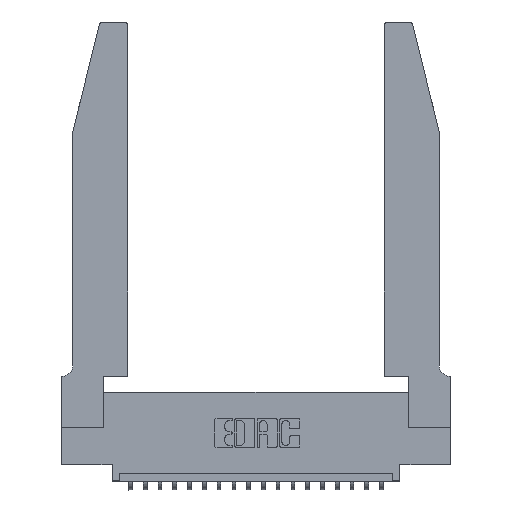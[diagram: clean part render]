
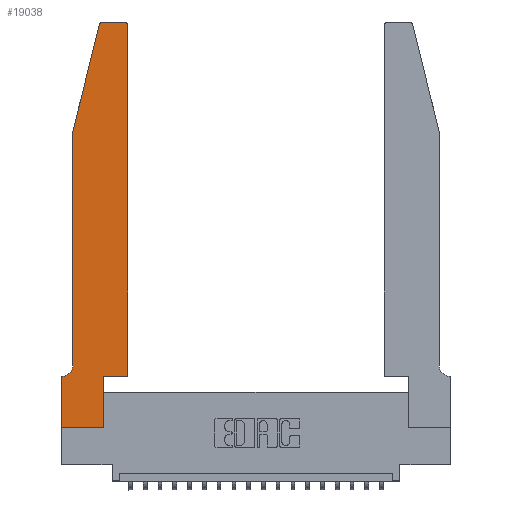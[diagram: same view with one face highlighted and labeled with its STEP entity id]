
A CAD part, top view. The second image highlights one B-rep face of the part: STEP entity #19038.
In plain terms, the highlighted planar face has unit normal (0, 0, 1).
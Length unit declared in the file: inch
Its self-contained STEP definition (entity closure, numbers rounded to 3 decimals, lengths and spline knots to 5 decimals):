
#1 = EDGE_CURVE ( 'NONE', #4615, #11518, #21165, .T. ) ;
#22 = CARTESIAN_POINT ( 'NONE',  ( 0.0755, 0.42, 0.37 ) ) ;
#1192 = DIRECTION ( 'NONE',  ( 1., 0., 0. ) ) ;
#1444 = CARTESIAN_POINT ( 'NONE',  ( 0., 0., 0.37 ) ) ;
#1651 = DIRECTION ( 'NONE',  ( 0., 0., 1. ) ) ;
#1704 = ORIENTED_EDGE ( 'NONE', *, *, #9884, .T. ) ;
#2663 = VECTOR ( 'NONE', #19163, 39.37008 ) ;
#2998 = CARTESIAN_POINT ( 'NONE',  ( 0.0755, 0.35, 0.37 ) ) ;
#3205 = DIRECTION ( 'NONE',  ( -1., 0., 0. ) ) ;
#3236 = EDGE_CURVE ( 'NONE', #10252, #7040, #8231, .T. ) ;
#3358 = CARTESIAN_POINT ( 'NONE',  ( 0., 0.35, 0.37 ) ) ;
#3461 = DIRECTION ( 'NONE',  ( 0., 0., 1. ) ) ;
#3543 = DIRECTION ( 'NONE',  ( 0., 0., 1. ) ) ;
#3619 = VERTEX_POINT ( 'NONE', #20377 ) ;
#4118 = AXIS2_PLACEMENT_3D ( 'NONE', #6324, #14975, #18029 ) ;
#4215 = VECTOR ( 'NONE', #3205, 39.37008 ) ;
#4345 = AXIS2_PLACEMENT_3D ( 'NONE', #15096, #3461, #5028 ) ;
#4615 = VERTEX_POINT ( 'NONE', #22 ) ;
#4709 = VERTEX_POINT ( 'NONE', #20488 ) ;
#4752 = DIRECTION ( 'NONE',  ( 0., -1., 0. ) ) ;
#4807 = ORIENTED_EDGE ( 'NONE', *, *, #6760, .T. ) ;
#5028 = DIRECTION ( 'NONE',  ( 1., 0., 0. ) ) ;
#5073 = DIRECTION ( 'NONE',  ( 1., 0., 0. ) ) ;
#5117 = ORIENTED_EDGE ( 'NONE', *, *, #3236, .T. ) ;
#5220 = VERTEX_POINT ( 'NONE', #20881 ) ;
#5966 = CARTESIAN_POINT ( 'NONE',  ( 0.2865, 0.35, 0.37 ) ) ;
#6016 = FACE_OUTER_BOUND ( 'NONE', #19877, .T. ) ;
#6113 = DIRECTION ( 'NONE',  ( 0., 1., 0. ) ) ;
#6208 = ORIENTED_EDGE ( 'NONE', *, *, #7324, .T. ) ;
#6324 = CARTESIAN_POINT ( 'NONE',  ( 0.0055, 0.42, 0.37 ) ) ;
#6427 = DIRECTION ( 'NONE',  ( -1., 0., 0. ) ) ;
#6599 = ORIENTED_EDGE ( 'NONE', *, *, #21737, .T. ) ;
#6621 = EDGE_CURVE ( 'NONE', #4709, #11150, #13332, .T. ) ;
#6627 = AXIS2_PLACEMENT_3D ( 'NONE', #8583, #3543, #20204 ) ;
#6760 = EDGE_CURVE ( 'NONE', #11150, #5220, #20127, .T. ) ;
#6766 = EDGE_CURVE ( 'NONE', #7576, #18585, #16740, .T. ) ;
#6931 = VECTOR ( 'NONE', #12697, 39.37008 ) ;
#7004 = VECTOR ( 'NONE', #1192, 39.37008 ) ;
#7040 = VERTEX_POINT ( 'NONE', #16041 ) ;
#7324 = EDGE_CURVE ( 'NONE', #18821, #4709, #19312, .T. ) ;
#7359 = LINE ( 'NONE', #5966, #11797 ) ;
#7439 = VECTOR ( 'NONE', #6427, 39.37008 ) ;
#7576 = VERTEX_POINT ( 'NONE', #8082 ) ;
#7864 = CARTESIAN_POINT ( 'NONE',  ( 0.4505, 0.35, 0.37 ) ) ;
#8082 = CARTESIAN_POINT ( 'NONE',  ( 0.284, 2.75, 0.37 ) ) ;
#8109 = VECTOR ( 'NONE', #14885, 39.37008 ) ;
#8231 = LINE ( 'NONE', #15295, #20787 ) ;
#8583 = CARTESIAN_POINT ( 'NONE',  ( 0.284, 2.72, 0.37 ) ) ;
#8804 = CARTESIAN_POINT ( 'NONE',  ( 0.4505, 2.72, 0.37 ) ) ;
#9005 = EDGE_CURVE ( 'NONE', #17906, #4615, #20296, .T. ) ;
#9147 = VECTOR ( 'NONE', #4752, 39.37008 ) ;
#9220 = CARTESIAN_POINT ( 'NONE',  ( 0.0755, 2., 0.37 ) ) ;
#9360 = CARTESIAN_POINT ( 'NONE',  ( 0.2865, 0.35, 0.37 ) ) ;
#9392 = LINE ( 'NONE', #18088, #9147 ) ;
#9553 = LINE ( 'NONE', #9220, #2663 ) ;
#9884 = EDGE_CURVE ( 'NONE', #5220, #7576, #21560, .T. ) ;
#10252 = VERTEX_POINT ( 'NONE', #1444 ) ;
#11150 = VERTEX_POINT ( 'NONE', #8804 ) ;
#11518 = VERTEX_POINT ( 'NONE', #20855 ) ;
#11589 = ORIENTED_EDGE ( 'NONE', *, *, #9005, .T. ) ;
#11640 = EDGE_CURVE ( 'NONE', #7040, #18821, #7359, .T. ) ;
#11797 = VECTOR ( 'NONE', #6113, 39.37008 ) ;
#12556 = CARTESIAN_POINT ( 'NONE',  ( 0.0755, 2., 0.37 ) ) ;
#12673 = LINE ( 'NONE', #2998, #7439 ) ;
#12697 = DIRECTION ( 'NONE',  ( 0., -1., 0. ) ) ;
#13332 = LINE ( 'NONE', #15124, #8109 ) ;
#13457 = DIRECTION ( 'NONE',  ( 1., 0., 0. ) ) ;
#13645 = ORIENTED_EDGE ( 'NONE', *, *, #6621, .T. ) ;
#13855 = CARTESIAN_POINT ( 'NONE',  ( 0.25487, 2.72718, 0.37 ) ) ;
#13914 = ORIENTED_EDGE ( 'NONE', *, *, #19600, .T. ) ;
#14885 = DIRECTION ( 'NONE',  ( 0., 1., 0. ) ) ;
#14975 = DIRECTION ( 'NONE',  ( 0., 0., -1. ) ) ;
#15064 = PLANE ( 'NONE',  #21667 ) ;
#15096 = CARTESIAN_POINT ( 'NONE',  ( 0.4205, 2.72, 0.37 ) ) ;
#15124 = CARTESIAN_POINT ( 'NONE',  ( 0.4505, 0.35, 0.37 ) ) ;
#15138 = CARTESIAN_POINT ( 'NONE',  ( 0.2605, 2.75, 0.37 ) ) ;
#15295 = CARTESIAN_POINT ( 'NONE',  ( 0., 0., 0.37 ) ) ;
#15922 = ORIENTED_EDGE ( 'NONE', *, *, #11640, .T. ) ;
#16041 = CARTESIAN_POINT ( 'NONE',  ( 0.2865, 0., 0.37 ) ) ;
#16740 = CIRCLE ( 'NONE', #6627, 0.03 ) ;
#16782 = EDGE_CURVE ( 'NONE', #11518, #3619, #12673, .T. ) ;
#17906 = VERTEX_POINT ( 'NONE', #18620 ) ;
#18029 = DIRECTION ( 'NONE',  ( -1., 0., 0. ) ) ;
#18088 = CARTESIAN_POINT ( 'NONE',  ( 0., 0., 0.37 ) ) ;
#18348 = ORIENTED_EDGE ( 'NONE', *, *, #16782, .T. ) ;
#18585 = VERTEX_POINT ( 'NONE', #13855 ) ;
#18620 = CARTESIAN_POINT ( 'NONE',  ( 0.0755, 2., 0.37 ) ) ;
#18821 = VERTEX_POINT ( 'NONE', #9360 ) ;
#19038 = ADVANCED_FACE ( 'NONE', ( #6016 ), #15064, .T. ) ;
#19163 = DIRECTION ( 'NONE',  ( -0.239, -0.971, 0. ) ) ;
#19312 = LINE ( 'NONE', #7864, #7004 ) ;
#19600 = EDGE_CURVE ( 'NONE', #3619, #10252, #9392, .T. ) ;
#19877 = EDGE_LOOP ( 'NONE', ( #1704, #21206, #6599, #11589, #21777, #18348, #13914, #5117, #15922, #6208, #13645, #4807 ) ) ;
#20127 = CIRCLE ( 'NONE', #4345, 0.03 ) ;
#20204 = DIRECTION ( 'NONE',  ( 1., 0., 0. ) ) ;
#20296 = LINE ( 'NONE', #12556, #6931 ) ;
#20377 = CARTESIAN_POINT ( 'NONE',  ( 0., 0.35, 0.37 ) ) ;
#20488 = CARTESIAN_POINT ( 'NONE',  ( 0.4505, 0.35, 0.37 ) ) ;
#20787 = VECTOR ( 'NONE', #5073, 39.37008 ) ;
#20855 = CARTESIAN_POINT ( 'NONE',  ( 0.0055, 0.35, 0.37 ) ) ;
#20881 = CARTESIAN_POINT ( 'NONE',  ( 0.4205, 2.75, 0.37 ) ) ;
#21165 = CIRCLE ( 'NONE', #4118, 0.07 ) ;
#21206 = ORIENTED_EDGE ( 'NONE', *, *, #6766, .T. ) ;
#21560 = LINE ( 'NONE', #15138, #4215 ) ;
#21667 = AXIS2_PLACEMENT_3D ( 'NONE', #3358, #1651, #13457 ) ;
#21737 = EDGE_CURVE ( 'NONE', #18585, #17906, #9553, .T. ) ;
#21777 = ORIENTED_EDGE ( 'NONE', *, *, #1, .T. ) ;
